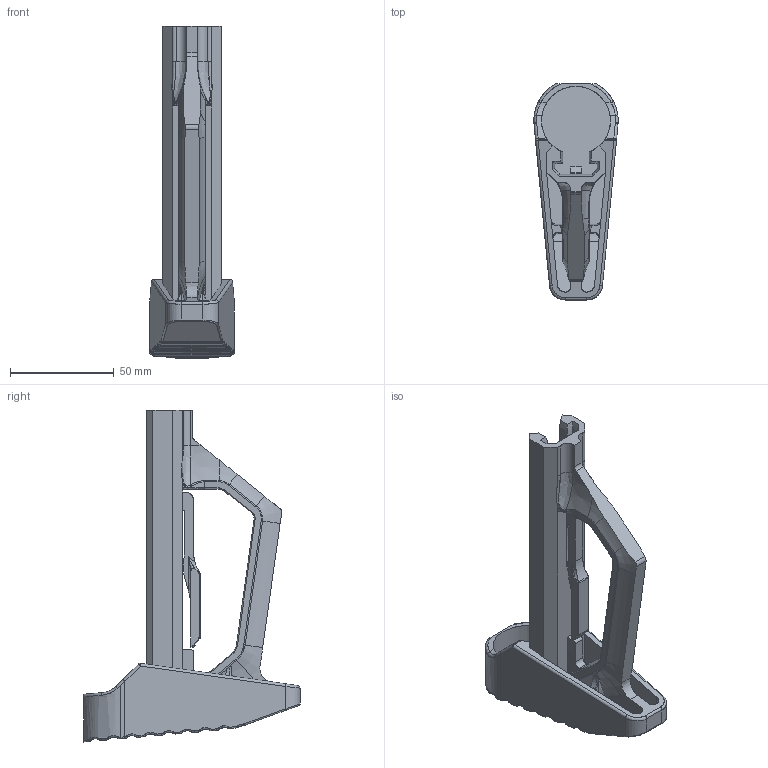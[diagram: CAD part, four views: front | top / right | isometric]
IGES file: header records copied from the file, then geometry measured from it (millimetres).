
Start section: SolidWorks IGES file using analytic representation for surfaces
Global section: file name: MKIIb Stock.IGS; native system: SolidWorks 2012; preprocessor: SolidWorks 2012; author: Pld; date: 130926.052127; units: inch
Bounding box: 40.64 x 104.14 x 160.02 mm (x, y, z)
Surface area: 44118 mm2 (no closed solid volume)
Topology: 0 solids, 0 shells, 372 faces, 3284 edges, 3279 vertices
Faces by surface type: bspline 212, revolution 160
